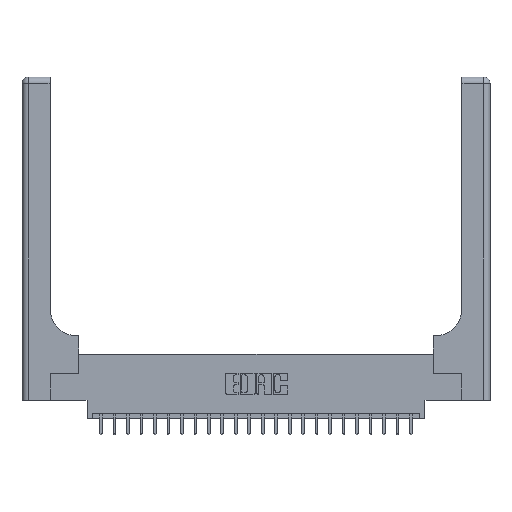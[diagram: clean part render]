
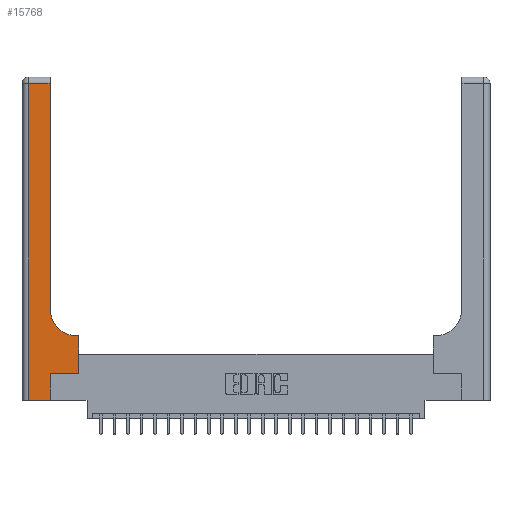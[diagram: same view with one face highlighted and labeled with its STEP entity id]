
A CAD part, top view. The second image highlights one B-rep face of the part: STEP entity #15768.
In plain terms, the highlighted planar face has unit normal (0, 0, 1).
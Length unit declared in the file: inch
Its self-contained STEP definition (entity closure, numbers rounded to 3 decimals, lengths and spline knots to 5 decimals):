
#111 = CARTESIAN_POINT ( 'NONE',  ( 0.26, 2.94, 0.37 ) ) ;
#997 = LINE ( 'NONE', #13680, #14536 ) ;
#1214 = EDGE_CURVE ( 'NONE', #5817, #18195, #11076, .T. ) ;
#2129 = EDGE_CURVE ( 'NONE', #18195, #10859, #9103, .T. ) ;
#2500 = EDGE_CURVE ( 'NONE', #15393, #10183, #19115, .T. ) ;
#2910 = DIRECTION ( 'NONE',  ( 1., 0., 0. ) ) ;
#2993 = VECTOR ( 'NONE', #9259, 39.37008 ) ;
#3541 = ORIENTED_EDGE ( 'NONE', *, *, #18851, .T. ) ;
#3607 = LINE ( 'NONE', #5537, #20604 ) ;
#3851 = EDGE_CURVE ( 'NONE', #17058, #20529, #997, .T. ) ;
#4031 = EDGE_CURVE ( 'NONE', #10859, #19405, #22485, .T. ) ;
#4096 = CARTESIAN_POINT ( 'NONE',  ( 0., 3., 0.37 ) ) ;
#4119 = DIRECTION ( 'NONE',  ( -1., 0., 0. ) ) ;
#4225 = DIRECTION ( 'NONE',  ( -1., 0., 0. ) ) ;
#4478 = CARTESIAN_POINT ( 'NONE',  ( 0.26, 0.85, 0.37 ) ) ;
#4954 = ORIENTED_EDGE ( 'NONE', *, *, #2129, .T. ) ;
#5475 = CARTESIAN_POINT ( 'NONE',  ( 0.528, 0.25, 0.37 ) ) ;
#5537 = CARTESIAN_POINT ( 'NONE',  ( 0.06, 3., 0.37 ) ) ;
#5539 = CARTESIAN_POINT ( 'NONE',  ( 0.265, 0., 0.37 ) ) ;
#5609 = AXIS2_PLACEMENT_3D ( 'NONE', #4096, #9671, #20651 ) ;
#5817 = VERTEX_POINT ( 'NONE', #6993 ) ;
#6993 = CARTESIAN_POINT ( 'NONE',  ( 0.265, 0.25, 0.37 ) ) ;
#7263 = VERTEX_POINT ( 'NONE', #14615 ) ;
#7460 = ORIENTED_EDGE ( 'NONE', *, *, #19894, .T. ) ;
#7706 = ORIENTED_EDGE ( 'NONE', *, *, #2500, .T. ) ;
#8273 = CARTESIAN_POINT ( 'NONE',  ( 0.51, 0.6, 0.37 ) ) ;
#8977 = CARTESIAN_POINT ( 'NONE',  ( 0.528, 0.25, 0.37 ) ) ;
#9103 = LINE ( 'NONE', #8977, #21120 ) ;
#9259 = DIRECTION ( 'NONE',  ( 1., 0., 0. ) ) ;
#9671 = DIRECTION ( 'NONE',  ( 0., 0., -1. ) ) ;
#10173 = DIRECTION ( 'NONE',  ( 0., 1., 0. ) ) ;
#10183 = VERTEX_POINT ( 'NONE', #111 ) ;
#10552 = DIRECTION ( 'NONE',  ( 1., 0., 0. ) ) ;
#10859 = VERTEX_POINT ( 'NONE', #22740 ) ;
#10942 = DIRECTION ( 'NONE',  ( 0., 1., 0. ) ) ;
#11076 = LINE ( 'NONE', #18435, #2993 ) ;
#11100 = CIRCLE ( 'NONE', #16893, 0.25 ) ;
#11182 = CARTESIAN_POINT ( 'NONE',  ( 0.265, 0., 0.37 ) ) ;
#11758 = VECTOR ( 'NONE', #10942, 39.37008 ) ;
#11923 = ORIENTED_EDGE ( 'NONE', *, *, #14455, .T. ) ;
#12922 = DIRECTION ( 'NONE',  ( 0., -1., 0. ) ) ;
#13680 = CARTESIAN_POINT ( 'NONE',  ( 0., 0., 0.37 ) ) ;
#14055 = CARTESIAN_POINT ( 'NONE',  ( 0.51, 0.85, 0.37 ) ) ;
#14211 = ORIENTED_EDGE ( 'NONE', *, *, #1214, .T. ) ;
#14455 = EDGE_CURVE ( 'NONE', #7263, #17058, #3607, .T. ) ;
#14525 = VECTOR ( 'NONE', #4119, 39.37008 ) ;
#14536 = VECTOR ( 'NONE', #2910, 39.37008 ) ;
#14615 = CARTESIAN_POINT ( 'NONE',  ( 0.06, 2.94, 0.37 ) ) ;
#15241 = CARTESIAN_POINT ( 'NONE',  ( 0.06, 0., 0.37 ) ) ;
#15393 = VERTEX_POINT ( 'NONE', #4478 ) ;
#15768 = ADVANCED_FACE ( 'NONE', ( #16920 ), #17145, .F. ) ;
#16117 = DIRECTION ( 'NONE',  ( 0., 1., 0. ) ) ;
#16457 = EDGE_CURVE ( 'NONE', #20529, #5817, #20231, .T. ) ;
#16680 = CARTESIAN_POINT ( 'NONE',  ( 0.26, 0.6, 0.37 ) ) ;
#16893 = AXIS2_PLACEMENT_3D ( 'NONE', #14055, #21427, #10552 ) ;
#16920 = FACE_OUTER_BOUND ( 'NONE', #22026, .T. ) ;
#16938 = CARTESIAN_POINT ( 'NONE',  ( 0., 2.94, 0.37 ) ) ;
#17058 = VERTEX_POINT ( 'NONE', #15241 ) ;
#17145 = PLANE ( 'NONE',  #5609 ) ;
#18195 = VERTEX_POINT ( 'NONE', #5475 ) ;
#18435 = CARTESIAN_POINT ( 'NONE',  ( 0.265, 0.25, 0.37 ) ) ;
#18851 = EDGE_CURVE ( 'NONE', #10183, #7263, #23187, .T. ) ;
#19115 = LINE ( 'NONE', #19598, #19972 ) ;
#19405 = VERTEX_POINT ( 'NONE', #8273 ) ;
#19598 = CARTESIAN_POINT ( 'NONE',  ( 0.26, 3., 0.37 ) ) ;
#19894 = EDGE_CURVE ( 'NONE', #19405, #15393, #11100, .T. ) ;
#19972 = VECTOR ( 'NONE', #10173, 39.37008 ) ;
#20117 = ORIENTED_EDGE ( 'NONE', *, *, #16457, .T. ) ;
#20231 = LINE ( 'NONE', #11182, #11758 ) ;
#20529 = VERTEX_POINT ( 'NONE', #5539 ) ;
#20604 = VECTOR ( 'NONE', #12922, 39.37008 ) ;
#20651 = DIRECTION ( 'NONE',  ( -1., 0., 0. ) ) ;
#21120 = VECTOR ( 'NONE', #16117, 39.37008 ) ;
#21427 = DIRECTION ( 'NONE',  ( 0., 0., -1. ) ) ;
#21459 = ORIENTED_EDGE ( 'NONE', *, *, #3851, .T. ) ;
#21872 = VECTOR ( 'NONE', #4225, 39.37008 ) ;
#22026 = EDGE_LOOP ( 'NONE', ( #7706, #3541, #11923, #21459, #20117, #14211, #4954, #22503, #7460 ) ) ;
#22485 = LINE ( 'NONE', #16680, #21872 ) ;
#22503 = ORIENTED_EDGE ( 'NONE', *, *, #4031, .T. ) ;
#22740 = CARTESIAN_POINT ( 'NONE',  ( 0.528, 0.6, 0.37 ) ) ;
#23187 = LINE ( 'NONE', #16938, #14525 ) ;
